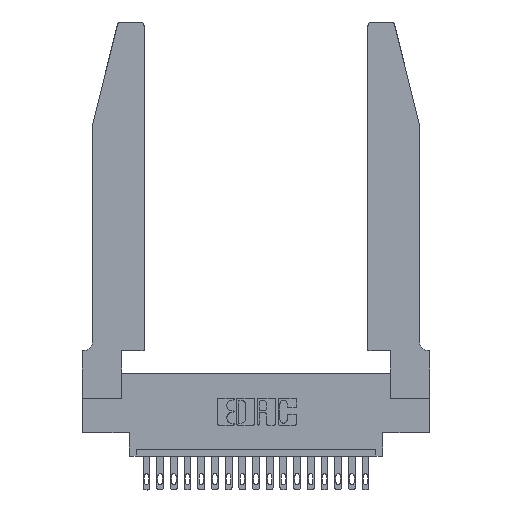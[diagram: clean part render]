
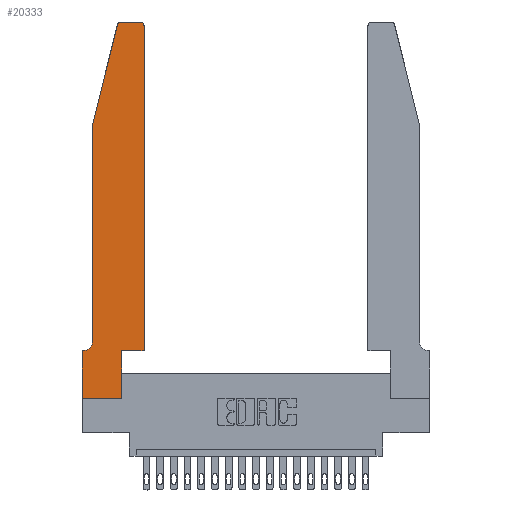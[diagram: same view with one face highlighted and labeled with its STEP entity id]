
A CAD part, top view. The second image highlights one B-rep face of the part: STEP entity #20333.
In plain terms, the highlighted planar face has unit normal (0, 0, 1).
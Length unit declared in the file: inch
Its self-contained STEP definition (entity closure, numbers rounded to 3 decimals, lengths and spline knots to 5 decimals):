
#316 = CARTESIAN_POINT ( 'NONE',  ( 0.2865, 0.35, 0.37 ) ) ;
#479 = VERTEX_POINT ( 'NONE', #18911 ) ;
#720 = EDGE_CURVE ( 'NONE', #8858, #17783, #12436, .T. ) ;
#798 = CARTESIAN_POINT ( 'NONE',  ( 0.0055, 0.42, 0.37 ) ) ;
#834 = CARTESIAN_POINT ( 'NONE',  ( 0.0755, 2., 0.37 ) ) ;
#886 = VERTEX_POINT ( 'NONE', #14772 ) ;
#898 = VERTEX_POINT ( 'NONE', #1616 ) ;
#928 = CARTESIAN_POINT ( 'NONE',  ( 0.4505, 0.35, 0.37 ) ) ;
#1616 = CARTESIAN_POINT ( 'NONE',  ( 0.4205, 2.75, 0.37 ) ) ;
#1677 = DIRECTION ( 'NONE',  ( 0., 0., 1. ) ) ;
#1800 = LINE ( 'NONE', #316, #11675 ) ;
#1892 = CARTESIAN_POINT ( 'NONE',  ( 0.284, 2.72, 0.37 ) ) ;
#2431 = ORIENTED_EDGE ( 'NONE', *, *, #9163, .T. ) ;
#2476 = CARTESIAN_POINT ( 'NONE',  ( 0.0055, 0.35, 0.37 ) ) ;
#2611 = VERTEX_POINT ( 'NONE', #19693 ) ;
#2623 = LINE ( 'NONE', #13560, #4651 ) ;
#2989 = EDGE_CURVE ( 'NONE', #898, #18582, #19189, .T. ) ;
#3028 = AXIS2_PLACEMENT_3D ( 'NONE', #20375, #5832, #20514 ) ;
#3277 = ORIENTED_EDGE ( 'NONE', *, *, #2989, .T. ) ;
#3428 = DIRECTION ( 'NONE',  ( 1., 0., 0. ) ) ;
#3627 = DIRECTION ( 'NONE',  ( 0., 1., 0. ) ) ;
#3820 = DIRECTION ( 'NONE',  ( 0., -1., 0. ) ) ;
#3829 = ORIENTED_EDGE ( 'NONE', *, *, #7328, .T. ) ;
#4060 = EDGE_CURVE ( 'NONE', #13520, #7774, #1800, .T. ) ;
#4098 = VECTOR ( 'NONE', #14096, 39.37008 ) ;
#4128 = AXIS2_PLACEMENT_3D ( 'NONE', #1892, #1677, #3428 ) ;
#4651 = VECTOR ( 'NONE', #20301, 39.37008 ) ;
#4804 = ORIENTED_EDGE ( 'NONE', *, *, #13561, .T. ) ;
#5110 = LINE ( 'NONE', #928, #4098 ) ;
#5263 = CARTESIAN_POINT ( 'NONE',  ( 0., 0., 0.37 ) ) ;
#5345 = AXIS2_PLACEMENT_3D ( 'NONE', #17429, #10892, #12442 ) ;
#5678 = DIRECTION ( 'NONE',  ( 0., 0., -1. ) ) ;
#5832 = DIRECTION ( 'NONE',  ( 0., 0., 1. ) ) ;
#5894 = VECTOR ( 'NONE', #13791, 39.37008 ) ;
#6143 = DIRECTION ( 'NONE',  ( 0., 1., 0. ) ) ;
#6252 = FACE_OUTER_BOUND ( 'NONE', #16663, .T. ) ;
#6365 = ORIENTED_EDGE ( 'NONE', *, *, #9011, .T. ) ;
#6635 = VECTOR ( 'NONE', #19943, 39.37008 ) ;
#7021 = VERTEX_POINT ( 'NONE', #834 ) ;
#7063 = LINE ( 'NONE', #9345, #19507 ) ;
#7328 = EDGE_CURVE ( 'NONE', #16576, #2611, #18409, .T. ) ;
#7774 = VERTEX_POINT ( 'NONE', #14668 ) ;
#7790 = CIRCLE ( 'NONE', #5345, 0.03 ) ;
#8184 = DIRECTION ( 'NONE',  ( -1., 0., 0. ) ) ;
#8658 = EDGE_CURVE ( 'NONE', #7021, #8858, #15548, .T. ) ;
#8858 = VERTEX_POINT ( 'NONE', #11635 ) ;
#9011 = EDGE_CURVE ( 'NONE', #886, #16345, #9964, .T. ) ;
#9163 = EDGE_CURVE ( 'NONE', #7774, #16576, #5110, .T. ) ;
#9345 = CARTESIAN_POINT ( 'NONE',  ( 0., 0., 0.37 ) ) ;
#9386 = CARTESIAN_POINT ( 'NONE',  ( 0., 0., 0.37 ) ) ;
#9820 = EDGE_CURVE ( 'NONE', #479, #7021, #10961, .T. ) ;
#9964 = LINE ( 'NONE', #9386, #17580 ) ;
#10892 = DIRECTION ( 'NONE',  ( 0., 0., 1. ) ) ;
#10961 = LINE ( 'NONE', #19872, #6635 ) ;
#11426 = CARTESIAN_POINT ( 'NONE',  ( 0.2605, 2.75, 0.37 ) ) ;
#11520 = EDGE_CURVE ( 'NONE', #2611, #898, #7790, .T. ) ;
#11526 = VECTOR ( 'NONE', #6143, 39.37008 ) ;
#11635 = CARTESIAN_POINT ( 'NONE',  ( 0.0755, 0.42, 0.37 ) ) ;
#11675 = VECTOR ( 'NONE', #3627, 39.37008 ) ;
#11754 = EDGE_CURVE ( 'NONE', #18582, #479, #20214, .T. ) ;
#12207 = DIRECTION ( 'NONE',  ( -1., 0., 0. ) ) ;
#12436 = CIRCLE ( 'NONE', #15194, 0.07 ) ;
#12442 = DIRECTION ( 'NONE',  ( 1., 0., 0. ) ) ;
#12573 = PLANE ( 'NONE',  #3028 ) ;
#12598 = CARTESIAN_POINT ( 'NONE',  ( 0.4505, 0.35, 0.37 ) ) ;
#13520 = VERTEX_POINT ( 'NONE', #15052 ) ;
#13560 = CARTESIAN_POINT ( 'NONE',  ( 0.0755, 0.35, 0.37 ) ) ;
#13561 = EDGE_CURVE ( 'NONE', #17783, #886, #2623, .T. ) ;
#13791 = DIRECTION ( 'NONE',  ( 0., -1., 0. ) ) ;
#14096 = DIRECTION ( 'NONE',  ( 1., 0., 0. ) ) ;
#14111 = ORIENTED_EDGE ( 'NONE', *, *, #4060, .T. ) ;
#14668 = CARTESIAN_POINT ( 'NONE',  ( 0.2865, 0.35, 0.37 ) ) ;
#14772 = CARTESIAN_POINT ( 'NONE',  ( 0., 0.35, 0.37 ) ) ;
#15052 = CARTESIAN_POINT ( 'NONE',  ( 0.2865, 0., 0.37 ) ) ;
#15194 = AXIS2_PLACEMENT_3D ( 'NONE', #798, #5678, #12207 ) ;
#15495 = ORIENTED_EDGE ( 'NONE', *, *, #9820, .T. ) ;
#15548 = LINE ( 'NONE', #18778, #5894 ) ;
#15611 = ORIENTED_EDGE ( 'NONE', *, *, #720, .T. ) ;
#16202 = CARTESIAN_POINT ( 'NONE',  ( 0.284, 2.75, 0.37 ) ) ;
#16345 = VERTEX_POINT ( 'NONE', #5263 ) ;
#16576 = VERTEX_POINT ( 'NONE', #17401 ) ;
#16663 = EDGE_LOOP ( 'NONE', ( #3277, #21004, #15495, #17856, #15611, #4804, #6365, #19646, #14111, #2431, #3829, #17638 ) ) ;
#17401 = CARTESIAN_POINT ( 'NONE',  ( 0.4505, 0.35, 0.37 ) ) ;
#17426 = VECTOR ( 'NONE', #8184, 39.37008 ) ;
#17429 = CARTESIAN_POINT ( 'NONE',  ( 0.4205, 2.72, 0.37 ) ) ;
#17517 = DIRECTION ( 'NONE',  ( 1., 0., 0. ) ) ;
#17580 = VECTOR ( 'NONE', #3820, 39.37008 ) ;
#17638 = ORIENTED_EDGE ( 'NONE', *, *, #11520, .T. ) ;
#17783 = VERTEX_POINT ( 'NONE', #2476 ) ;
#17856 = ORIENTED_EDGE ( 'NONE', *, *, #8658, .T. ) ;
#18409 = LINE ( 'NONE', #12598, #11526 ) ;
#18582 = VERTEX_POINT ( 'NONE', #16202 ) ;
#18778 = CARTESIAN_POINT ( 'NONE',  ( 0.0755, 2., 0.37 ) ) ;
#18911 = CARTESIAN_POINT ( 'NONE',  ( 0.25487, 2.72718, 0.37 ) ) ;
#19189 = LINE ( 'NONE', #11426, #17426 ) ;
#19507 = VECTOR ( 'NONE', #17517, 39.37008 ) ;
#19514 = EDGE_CURVE ( 'NONE', #16345, #13520, #7063, .T. ) ;
#19646 = ORIENTED_EDGE ( 'NONE', *, *, #19514, .T. ) ;
#19693 = CARTESIAN_POINT ( 'NONE',  ( 0.4505, 2.72, 0.37 ) ) ;
#19872 = CARTESIAN_POINT ( 'NONE',  ( 0.0755, 2., 0.37 ) ) ;
#19943 = DIRECTION ( 'NONE',  ( -0.239, -0.971, 0. ) ) ;
#20214 = CIRCLE ( 'NONE', #4128, 0.03 ) ;
#20301 = DIRECTION ( 'NONE',  ( -1., 0., 0. ) ) ;
#20333 = ADVANCED_FACE ( 'NONE', ( #6252 ), #12573, .T. ) ;
#20375 = CARTESIAN_POINT ( 'NONE',  ( 0., 0.35, 0.37 ) ) ;
#20514 = DIRECTION ( 'NONE',  ( 1., 0., 0. ) ) ;
#21004 = ORIENTED_EDGE ( 'NONE', *, *, #11754, .T. ) ;
